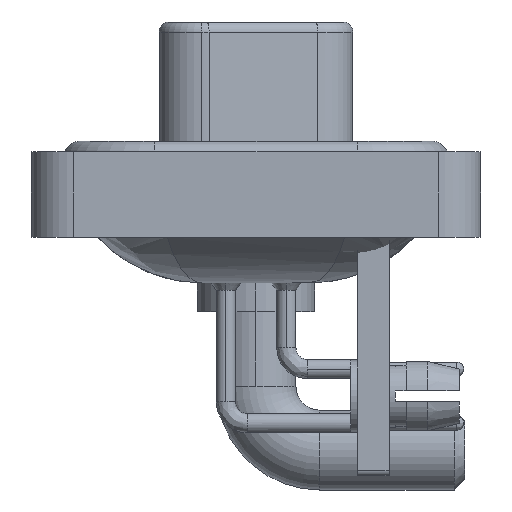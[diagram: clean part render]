
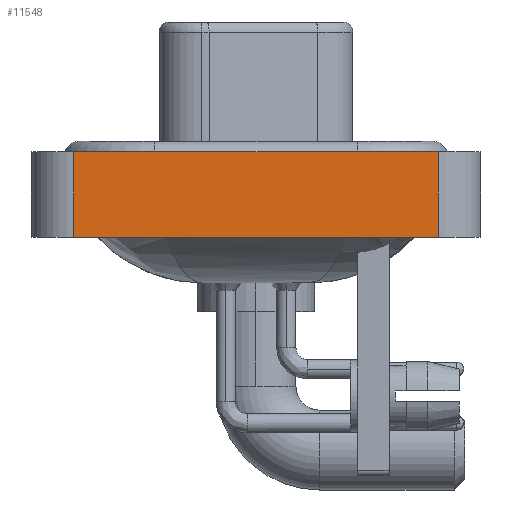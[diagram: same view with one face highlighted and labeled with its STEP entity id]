
A CAD part, left-side view. The second image highlights one B-rep face of the part: STEP entity #11548.
In plain terms, the highlighted planar face has unit normal (-1, 0, 0).
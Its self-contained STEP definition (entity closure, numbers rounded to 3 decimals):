
#607 = LINE ( 'NONE', #3352, #1842 ) ;
#1842 = VECTOR ( 'NONE', #3669, 1000. ) ;
#1849 = CARTESIAN_POINT ( 'NONE',  ( -7.35, -8.55, -3.6 ) ) ;
#3352 = CARTESIAN_POINT ( 'NONE',  ( -7.35, -8.55, -3.6 ) ) ;
#3383 = EDGE_CURVE ( 'NONE', #29224, #26435, #607, .T. ) ;
#3669 = DIRECTION ( 'NONE',  ( 0., 0., 1. ) ) ;
#4574 = DIRECTION ( 'NONE',  ( 0., 0., 1. ) ) ;
#4795 = DIRECTION ( 'NONE',  ( 0., -1., 0. ) ) ;
#7161 = DIRECTION ( 'NONE',  ( -1., 0., 0. ) ) ;
#7499 = CARTESIAN_POINT ( 'NONE',  ( -7.35, 8.55, 0.4 ) ) ;
#8681 = CARTESIAN_POINT ( 'NONE',  ( -7.35, 8.55, -3.6 ) ) ;
#9210 = EDGE_CURVE ( 'NONE', #16587, #29224, #14859, .T. ) ;
#9353 = EDGE_CURVE ( 'NONE', #20084, #26435, #10613, .T. ) ;
#10612 = VECTOR ( 'NONE', #15328, 1000. ) ;
#10613 = LINE ( 'NONE', #15476, #10612 ) ;
#11548 = ADVANCED_FACE ( 'NONE', ( #26726 ), #31410, .T. ) ;
#12740 = VECTOR ( 'NONE', #30251, 1000. ) ;
#13492 = CARTESIAN_POINT ( 'NONE',  ( -7.35, -8.55, 0.4 ) ) ;
#13561 = AXIS2_PLACEMENT_3D ( 'NONE', #28984, #7161, #4574 ) ;
#14016 = EDGE_CURVE ( 'NONE', #16587, #20084, #15719, .T. ) ;
#14859 = LINE ( 'NONE', #20171, #29618 ) ;
#14918 = ORIENTED_EDGE ( 'NONE', *, *, #14016, .F. ) ;
#15328 = DIRECTION ( 'NONE',  ( 0., -1., 0. ) ) ;
#15476 = CARTESIAN_POINT ( 'NONE',  ( -7.35, -8.55, 0.4 ) ) ;
#15719 = LINE ( 'NONE', #30086, #12740 ) ;
#16587 = VERTEX_POINT ( 'NONE', #8681 ) ;
#17526 = EDGE_LOOP ( 'NONE', ( #27940, #20117, #14918, #30247 ) ) ;
#20084 = VERTEX_POINT ( 'NONE', #7499 ) ;
#20117 = ORIENTED_EDGE ( 'NONE', *, *, #9353, .F. ) ;
#20171 = CARTESIAN_POINT ( 'NONE',  ( -7.35, -8.55, -3.6 ) ) ;
#26435 = VERTEX_POINT ( 'NONE', #13492 ) ;
#26726 = FACE_OUTER_BOUND ( 'NONE', #17526, .T. ) ;
#27940 = ORIENTED_EDGE ( 'NONE', *, *, #3383, .T. ) ;
#28984 = CARTESIAN_POINT ( 'NONE',  ( -7.35, -8.55, -3.6 ) ) ;
#29224 = VERTEX_POINT ( 'NONE', #1849 ) ;
#29618 = VECTOR ( 'NONE', #4795, 1000. ) ;
#30086 = CARTESIAN_POINT ( 'NONE',  ( -7.35, 8.55, -3.6 ) ) ;
#30247 = ORIENTED_EDGE ( 'NONE', *, *, #9210, .T. ) ;
#30251 = DIRECTION ( 'NONE',  ( 0., 0., 1. ) ) ;
#31410 = PLANE ( 'NONE',  #13561 ) ;
